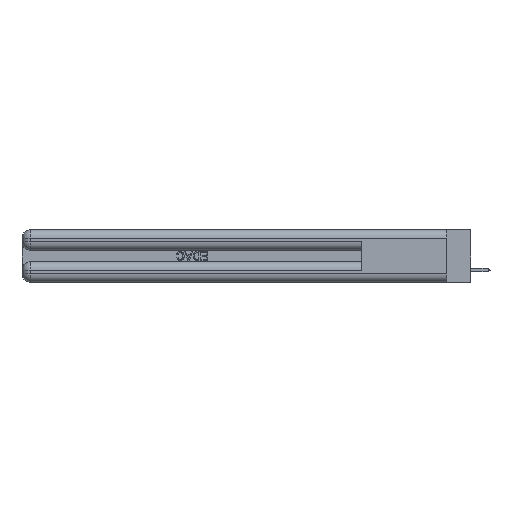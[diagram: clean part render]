
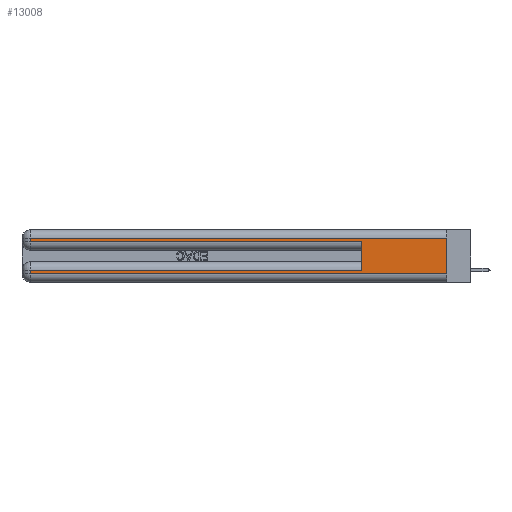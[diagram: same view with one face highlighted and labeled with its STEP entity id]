
A CAD part, left-side view. The second image highlights one B-rep face of the part: STEP entity #13008.
In plain terms, the highlighted planar face has unit normal (-1, 0, 0).
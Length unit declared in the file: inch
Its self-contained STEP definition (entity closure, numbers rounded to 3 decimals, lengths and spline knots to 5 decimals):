
#1266 = LINE ( 'NONE', #26376, #17011 ) ;
#1418 = VERTEX_POINT ( 'NONE', #13432 ) ;
#2089 = CARTESIAN_POINT ( 'NONE',  ( 0., 0., 0.285 ) ) ;
#2228 = DIRECTION ( 'NONE',  ( 0., 0., -1. ) ) ;
#2708 = VERTEX_POINT ( 'NONE', #29700 ) ;
#2787 = EDGE_CURVE ( 'NONE', #23645, #32976, #34346, .T. ) ;
#3220 = CARTESIAN_POINT ( 'NONE',  ( 0., 0., 0.06 ) ) ;
#3359 = CARTESIAN_POINT ( 'NONE',  ( 0., 0., 0.085 ) ) ;
#3573 = VECTOR ( 'NONE', #43606, 39.37008 ) ;
#3943 = CARTESIAN_POINT ( 'NONE',  ( 0., 0., 0.37 ) ) ;
#4719 = DIRECTION ( 'NONE',  ( 0., 1., 0. ) ) ;
#5212 = LINE ( 'NONE', #3359, #42153 ) ;
#5479 = FACE_OUTER_BOUND ( 'NONE', #29298, .T. ) ;
#5691 = DIRECTION ( 'NONE',  ( 0., 0., -1. ) ) ;
#6440 = ORIENTED_EDGE ( 'NONE', *, *, #21024, .T. ) ;
#7097 = VERTEX_POINT ( 'NONE', #19008 ) ;
#7298 = VECTOR ( 'NONE', #13047, 39.37008 ) ;
#7983 = EDGE_CURVE ( 'NONE', #13665, #23645, #26571, .T. ) ;
#9590 = EDGE_CURVE ( 'NONE', #7097, #24002, #5212, .T. ) ;
#10730 = LINE ( 'NONE', #3220, #44350 ) ;
#11204 = EDGE_CURVE ( 'NONE', #24002, #2708, #28501, .T. ) ;
#11803 = ORIENTED_EDGE ( 'NONE', *, *, #28788, .T. ) ;
#12257 = DIRECTION ( 'NONE',  ( 0., -1., 0. ) ) ;
#13008 = ADVANCED_FACE ( 'NONE', ( #5479 ), #38123, .F. ) ;
#13047 = DIRECTION ( 'NONE',  ( 0., 0., -1. ) ) ;
#13432 = CARTESIAN_POINT ( 'NONE',  ( 0., 0.6, 0.285 ) ) ;
#13665 = VERTEX_POINT ( 'NONE', #44280 ) ;
#15810 = VECTOR ( 'NONE', #5691, 39.37008 ) ;
#16224 = VECTOR ( 'NONE', #4719, 39.37008 ) ;
#16912 = CARTESIAN_POINT ( 'NONE',  ( 0., 2.94, 0.085 ) ) ;
#17011 = VECTOR ( 'NONE', #2228, 39.37008 ) ;
#17259 = AXIS2_PLACEMENT_3D ( 'NONE', #3943, #28234, #31755 ) ;
#18037 = CARTESIAN_POINT ( 'NONE',  ( 0., 0., 0.31 ) ) ;
#18755 = CARTESIAN_POINT ( 'NONE',  ( 0., 2.94, 0.31 ) ) ;
#19008 = CARTESIAN_POINT ( 'NONE',  ( 0., 0.6, 0.085 ) ) ;
#19743 = VECTOR ( 'NONE', #12257, 39.37008 ) ;
#21024 = EDGE_CURVE ( 'NONE', #2708, #29577, #10730, .T. ) ;
#21236 = DIRECTION ( 'NONE',  ( 0., 1., 0. ) ) ;
#23343 = CARTESIAN_POINT ( 'NONE',  ( 0., 2.94, 0.37 ) ) ;
#23405 = ORIENTED_EDGE ( 'NONE', *, *, #27728, .F. ) ;
#23549 = CARTESIAN_POINT ( 'NONE',  ( 0., 0., 0.06 ) ) ;
#23645 = VERTEX_POINT ( 'NONE', #18755 ) ;
#23823 = EDGE_CURVE ( 'NONE', #13665, #29577, #1266, .T. ) ;
#24002 = VERTEX_POINT ( 'NONE', #16912 ) ;
#25756 = ORIENTED_EDGE ( 'NONE', *, *, #9590, .T. ) ;
#25769 = CARTESIAN_POINT ( 'NONE',  ( 0., 2.94, 0.285 ) ) ;
#26376 = CARTESIAN_POINT ( 'NONE',  ( 0., 0., 0.37 ) ) ;
#26571 = LINE ( 'NONE', #18037, #16224 ) ;
#26628 = CARTESIAN_POINT ( 'NONE',  ( 0., 0.6, 0.145 ) ) ;
#27728 = EDGE_CURVE ( 'NONE', #7097, #1418, #35704, .T. ) ;
#28234 = DIRECTION ( 'NONE',  ( 1., 0., 0. ) ) ;
#28501 = LINE ( 'NONE', #23343, #7298 ) ;
#28788 = EDGE_CURVE ( 'NONE', #32976, #1418, #36702, .T. ) ;
#29298 = EDGE_LOOP ( 'NONE', ( #32726, #33278, #37424, #11803, #23405, #25756, #34843, #6440 ) ) ;
#29577 = VERTEX_POINT ( 'NONE', #23549 ) ;
#29700 = CARTESIAN_POINT ( 'NONE',  ( 0., 2.94, 0.06 ) ) ;
#29995 = CARTESIAN_POINT ( 'NONE',  ( 0., 2.94, 0.37 ) ) ;
#31755 = DIRECTION ( 'NONE',  ( 0., 0., -1. ) ) ;
#32726 = ORIENTED_EDGE ( 'NONE', *, *, #23823, .F. ) ;
#32976 = VERTEX_POINT ( 'NONE', #25769 ) ;
#33278 = ORIENTED_EDGE ( 'NONE', *, *, #7983, .T. ) ;
#34346 = LINE ( 'NONE', #29995, #15810 ) ;
#34523 = DIRECTION ( 'NONE',  ( 0., -1., 0. ) ) ;
#34843 = ORIENTED_EDGE ( 'NONE', *, *, #11204, .T. ) ;
#35704 = LINE ( 'NONE', #26628, #3573 ) ;
#36702 = LINE ( 'NONE', #2089, #19743 ) ;
#37424 = ORIENTED_EDGE ( 'NONE', *, *, #2787, .T. ) ;
#38123 = PLANE ( 'NONE',  #17259 ) ;
#42153 = VECTOR ( 'NONE', #21236, 39.37008 ) ;
#43606 = DIRECTION ( 'NONE',  ( 0., 0., 1. ) ) ;
#44280 = CARTESIAN_POINT ( 'NONE',  ( 0., 0., 0.31 ) ) ;
#44350 = VECTOR ( 'NONE', #34523, 39.37008 ) ;
